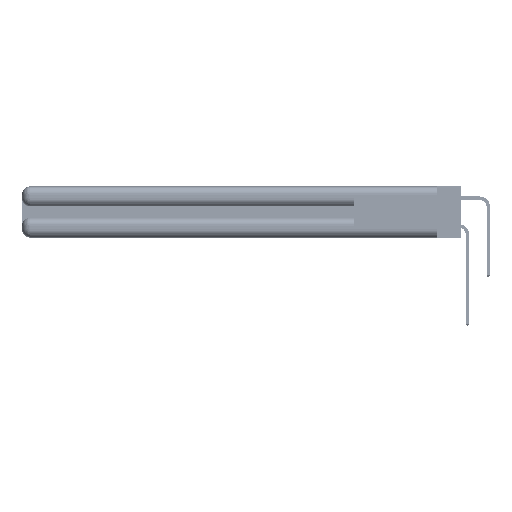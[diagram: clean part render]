
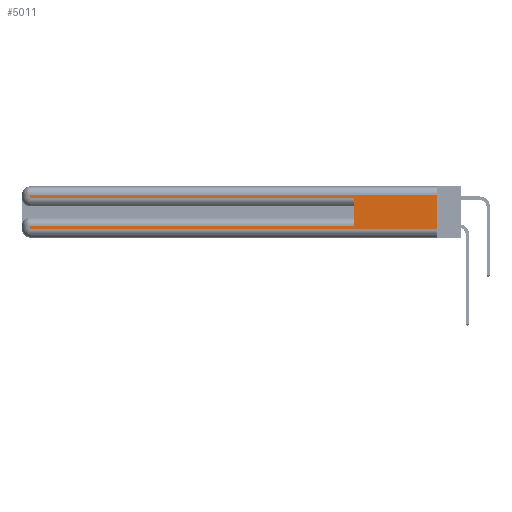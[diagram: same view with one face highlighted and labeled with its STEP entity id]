
A CAD part, left-side view. The second image highlights one B-rep face of the part: STEP entity #5011.
In plain terms, the highlighted planar face has unit normal (-1, 0, 0).
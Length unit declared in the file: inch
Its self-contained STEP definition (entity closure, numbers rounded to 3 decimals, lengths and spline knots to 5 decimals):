
#145 = ORIENTED_EDGE ( 'NONE', *, *, #7833, .F. ) ;
#299 = EDGE_CURVE ( 'NONE', #33043, #6974, #30735, .T. ) ;
#643 = CARTESIAN_POINT ( 'NONE',  ( 0., 0., 0.31 ) ) ;
#847 = LINE ( 'NONE', #14053, #35496 ) ;
#1968 = VERTEX_POINT ( 'NONE', #19359 ) ;
#2068 = CARTESIAN_POINT ( 'NONE',  ( 0., 0., 0.31 ) ) ;
#2267 = VECTOR ( 'NONE', #40305, 39.37008 ) ;
#2443 = ORIENTED_EDGE ( 'NONE', *, *, #26056, .T. ) ;
#5011 = ADVANCED_FACE ( 'NONE', ( #51041 ), #12280, .F. ) ;
#5233 = CARTESIAN_POINT ( 'NONE',  ( 0., 0., 0.085 ) ) ;
#5526 = CARTESIAN_POINT ( 'NONE',  ( 0., 2.94, 0.37 ) ) ;
#6974 = VERTEX_POINT ( 'NONE', #21778 ) ;
#7206 = EDGE_CURVE ( 'NONE', #43427, #14191, #847, .T. ) ;
#7407 = LINE ( 'NONE', #5526, #28665 ) ;
#7833 = EDGE_CURVE ( 'NONE', #33043, #28821, #36087, .T. ) ;
#11750 = CARTESIAN_POINT ( 'NONE',  ( 0., 0.6, 0.285 ) ) ;
#12112 = CARTESIAN_POINT ( 'NONE',  ( 0., 0., 0.06 ) ) ;
#12280 = PLANE ( 'NONE',  #27941 ) ;
#13315 = CARTESIAN_POINT ( 'NONE',  ( 0., 0., 0.285 ) ) ;
#14053 = CARTESIAN_POINT ( 'NONE',  ( 0., 0.6, 0.145 ) ) ;
#14191 = VERTEX_POINT ( 'NONE', #11750 ) ;
#14228 = DIRECTION ( 'NONE',  ( 0., 0., 1. ) ) ;
#14277 = CARTESIAN_POINT ( 'NONE',  ( 0., 2.94, 0.06 ) ) ;
#15138 = ORIENTED_EDGE ( 'NONE', *, *, #7206, .F. ) ;
#16633 = VECTOR ( 'NONE', #47344, 39.37008 ) ;
#16648 = DIRECTION ( 'NONE',  ( 0., -1., 0. ) ) ;
#17304 = VECTOR ( 'NONE', #38179, 39.37008 ) ;
#17399 = VECTOR ( 'NONE', #23442, 39.37008 ) ;
#17664 = DIRECTION ( 'NONE',  ( 0., 0., -1. ) ) ;
#18613 = VERTEX_POINT ( 'NONE', #14277 ) ;
#19359 = CARTESIAN_POINT ( 'NONE',  ( 0., 2.94, 0.085 ) ) ;
#21381 = CARTESIAN_POINT ( 'NONE',  ( 0., 0., 0.37 ) ) ;
#21778 = CARTESIAN_POINT ( 'NONE',  ( 0., 2.94, 0.31 ) ) ;
#22020 = CARTESIAN_POINT ( 'NONE',  ( 0., 0., 0.37 ) ) ;
#22787 = EDGE_LOOP ( 'NONE', ( #145, #38345, #32016, #51599, #15138, #55118, #2443, #57233 ) ) ;
#23335 = EDGE_CURVE ( 'NONE', #18613, #28821, #24005, .T. ) ;
#23442 = DIRECTION ( 'NONE',  ( 0., 1., 0. ) ) ;
#24005 = LINE ( 'NONE', #12112, #56831 ) ;
#24143 = VECTOR ( 'NONE', #17664, 39.37008 ) ;
#26056 = EDGE_CURVE ( 'NONE', #1968, #18613, #40602, .T. ) ;
#27941 = AXIS2_PLACEMENT_3D ( 'NONE', #21381, #57139, #30462 ) ;
#28665 = VECTOR ( 'NONE', #54982, 39.37008 ) ;
#28821 = VERTEX_POINT ( 'NONE', #55404 ) ;
#29448 = LINE ( 'NONE', #5233, #17399 ) ;
#30462 = DIRECTION ( 'NONE',  ( 0., 0., -1. ) ) ;
#30735 = LINE ( 'NONE', #2068, #17304 ) ;
#32016 = ORIENTED_EDGE ( 'NONE', *, *, #41879, .T. ) ;
#33043 = VERTEX_POINT ( 'NONE', #643 ) ;
#33427 = CARTESIAN_POINT ( 'NONE',  ( 0., 2.94, 0.285 ) ) ;
#33904 = CARTESIAN_POINT ( 'NONE',  ( 0., 2.94, 0.37 ) ) ;
#34506 = EDGE_CURVE ( 'NONE', #43427, #1968, #29448, .T. ) ;
#35496 = VECTOR ( 'NONE', #14228, 39.37008 ) ;
#36087 = LINE ( 'NONE', #22020, #24143 ) ;
#38179 = DIRECTION ( 'NONE',  ( 0., 1., 0. ) ) ;
#38345 = ORIENTED_EDGE ( 'NONE', *, *, #299, .T. ) ;
#40305 = DIRECTION ( 'NONE',  ( 0., -1., 0. ) ) ;
#40602 = LINE ( 'NONE', #33904, #16633 ) ;
#41879 = EDGE_CURVE ( 'NONE', #6974, #46707, #7407, .T. ) ;
#43427 = VERTEX_POINT ( 'NONE', #52867 ) ;
#46366 = EDGE_CURVE ( 'NONE', #46707, #14191, #50082, .T. ) ;
#46707 = VERTEX_POINT ( 'NONE', #33427 ) ;
#47344 = DIRECTION ( 'NONE',  ( 0., 0., -1. ) ) ;
#50082 = LINE ( 'NONE', #13315, #2267 ) ;
#51041 = FACE_OUTER_BOUND ( 'NONE', #22787, .T. ) ;
#51599 = ORIENTED_EDGE ( 'NONE', *, *, #46366, .T. ) ;
#52867 = CARTESIAN_POINT ( 'NONE',  ( 0., 0.6, 0.085 ) ) ;
#54982 = DIRECTION ( 'NONE',  ( 0., 0., -1. ) ) ;
#55118 = ORIENTED_EDGE ( 'NONE', *, *, #34506, .T. ) ;
#55404 = CARTESIAN_POINT ( 'NONE',  ( 0., 0., 0.06 ) ) ;
#56831 = VECTOR ( 'NONE', #16648, 39.37008 ) ;
#57139 = DIRECTION ( 'NONE',  ( 1., 0., 0. ) ) ;
#57233 = ORIENTED_EDGE ( 'NONE', *, *, #23335, .T. ) ;
